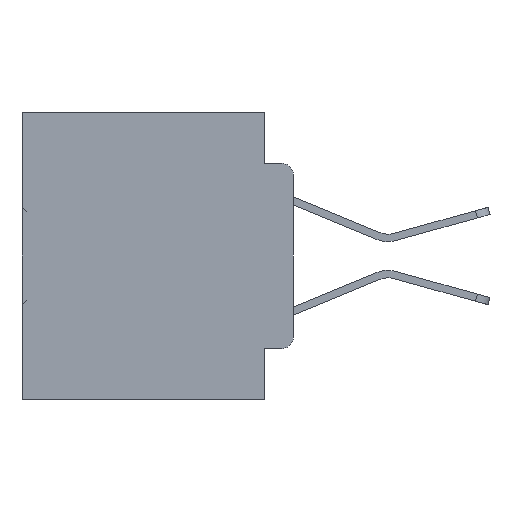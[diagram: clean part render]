
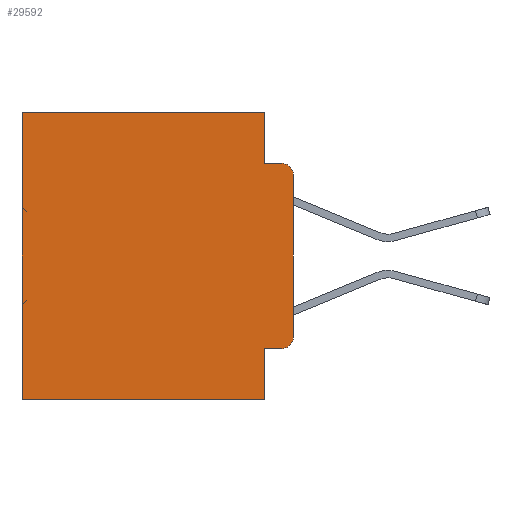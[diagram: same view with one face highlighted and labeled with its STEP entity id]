
A CAD part, left-side view. The second image highlights one B-rep face of the part: STEP entity #29592.
In plain terms, the highlighted planar face has unit normal (-1, 0, 0).
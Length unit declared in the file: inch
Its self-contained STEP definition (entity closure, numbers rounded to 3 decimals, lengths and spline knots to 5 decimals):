
#120 = DIRECTION ( 'NONE',  ( 0., 0., -1. ) ) ;
#474 = DIRECTION ( 'NONE',  ( 0., 1., 0. ) ) ;
#1241 = CARTESIAN_POINT ( 'NONE',  ( 0.298, 0.051, 0. ) ) ;
#1814 = CARTESIAN_POINT ( 'NONE',  ( 0.298, 0., 0. ) ) ;
#1868 = CARTESIAN_POINT ( 'NONE',  ( 0.298, 0.02, -0.3915 ) ) ;
#2194 = CIRCLE ( 'NONE', #7619, 0.02 ) ;
#2796 = EDGE_CURVE ( 'NONE', #21995, #24222, #34332, .T. ) ;
#3744 = LINE ( 'NONE', #35566, #21834 ) ;
#3917 = DIRECTION ( 'NONE',  ( 0., -1., 0. ) ) ;
#4084 = DIRECTION ( 'NONE',  ( -1., 0., 0. ) ) ;
#4510 = LINE ( 'NONE', #27494, #24777 ) ;
#5213 = CARTESIAN_POINT ( 'NONE',  ( 0.298, 0.473, 0. ) ) ;
#5308 = DIRECTION ( 'NONE',  ( 0., 0., -1. ) ) ;
#5920 = DIRECTION ( 'NONE',  ( 0., 1., 0. ) ) ;
#6884 = FACE_OUTER_BOUND ( 'NONE', #13854, .T. ) ;
#7331 = AXIS2_PLACEMENT_3D ( 'NONE', #1814, #30416, #13293 ) ;
#7619 = AXIS2_PLACEMENT_3D ( 'NONE', #15950, #4084, #36111 ) ;
#8648 = VERTEX_POINT ( 'NONE', #34553 ) ;
#11199 = CARTESIAN_POINT ( 'NONE',  ( 0.298, 0., -0.3915 ) ) ;
#11206 = EDGE_CURVE ( 'NONE', #33371, #8648, #17045, .T. ) ;
#11445 = CARTESIAN_POINT ( 'NONE',  ( 0.298, 0.051, -0.4115 ) ) ;
#11586 = EDGE_CURVE ( 'NONE', #36654, #33371, #28913, .T. ) ;
#12088 = ORIENTED_EDGE ( 'NONE', *, *, #11206, .T. ) ;
#12143 = ORIENTED_EDGE ( 'NONE', *, *, #11586, .T. ) ;
#12160 = VECTOR ( 'NONE', #5920, 39.37008 ) ;
#13293 = DIRECTION ( 'NONE',  ( 0., 0., -1. ) ) ;
#13363 = EDGE_CURVE ( 'NONE', #26483, #35936, #26423, .T. ) ;
#13854 = EDGE_LOOP ( 'NONE', ( #20688, #20316, #27046, #24259, #12143, #12088, #21964, #13902, #32856, #25086 ) ) ;
#13902 = ORIENTED_EDGE ( 'NONE', *, *, #2796, .F. ) ;
#14044 = CARTESIAN_POINT ( 'NONE',  ( 0.298, 0.473, 0. ) ) ;
#14551 = LINE ( 'NONE', #31704, #25005 ) ;
#14837 = VECTOR ( 'NONE', #34196, 39.37008 ) ;
#15950 = CARTESIAN_POINT ( 'NONE',  ( 0.298, 0.02, -0.1085 ) ) ;
#17043 = LINE ( 'NONE', #29102, #37125 ) ;
#17045 = LINE ( 'NONE', #14044, #14837 ) ;
#18146 = EDGE_CURVE ( 'NONE', #27950, #18705, #21348, .T. ) ;
#18705 = VERTEX_POINT ( 'NONE', #11199 ) ;
#19619 = VECTOR ( 'NONE', #28685, 39.37008 ) ;
#20316 = ORIENTED_EDGE ( 'NONE', *, *, #36227, .T. ) ;
#20688 = ORIENTED_EDGE ( 'NONE', *, *, #35152, .F. ) ;
#20869 = VECTOR ( 'NONE', #5308, 39.37008 ) ;
#21348 = CIRCLE ( 'NONE', #30350, 0.02 ) ;
#21834 = VECTOR ( 'NONE', #3917, 39.37008 ) ;
#21964 = ORIENTED_EDGE ( 'NONE', *, *, #29976, .F. ) ;
#21995 = VERTEX_POINT ( 'NONE', #11445 ) ;
#22677 = DIRECTION ( 'NONE',  ( 0., 0., -1. ) ) ;
#24222 = VERTEX_POINT ( 'NONE', #34350 ) ;
#24259 = ORIENTED_EDGE ( 'NONE', *, *, #35663, .F. ) ;
#24777 = VECTOR ( 'NONE', #474, 39.37008 ) ;
#25005 = VECTOR ( 'NONE', #22677, 39.37008 ) ;
#25086 = ORIENTED_EDGE ( 'NONE', *, *, #18146, .T. ) ;
#25589 = CARTESIAN_POINT ( 'NONE',  ( 0.298, 0.051, -0.0885 ) ) ;
#25859 = CARTESIAN_POINT ( 'NONE',  ( 0.298, 0.051, -0.0885 ) ) ;
#25896 = CARTESIAN_POINT ( 'NONE',  ( 0.298, 0., 0. ) ) ;
#26423 = LINE ( 'NONE', #25859, #19619 ) ;
#26483 = VERTEX_POINT ( 'NONE', #25589 ) ;
#27046 = ORIENTED_EDGE ( 'NONE', *, *, #13363, .F. ) ;
#27269 = DIRECTION ( 'NONE',  ( -1., 0., 0. ) ) ;
#27494 = CARTESIAN_POINT ( 'NONE',  ( 0.298, 0., -0.5 ) ) ;
#27648 = DIRECTION ( 'NONE',  ( 0., 0., -1. ) ) ;
#27950 = VERTEX_POINT ( 'NONE', #36681 ) ;
#28685 = DIRECTION ( 'NONE',  ( 0., -1., 0. ) ) ;
#28913 = LINE ( 'NONE', #25896, #12160 ) ;
#29102 = CARTESIAN_POINT ( 'NONE',  ( 0.298, 0., 0. ) ) ;
#29493 = PLANE ( 'NONE',  #7331 ) ;
#29592 = ADVANCED_FACE ( 'NONE', ( #6884 ), #29493, .F. ) ;
#29720 = CARTESIAN_POINT ( 'NONE',  ( 0.298, 0., -0.1085 ) ) ;
#29976 = EDGE_CURVE ( 'NONE', #24222, #8648, #4510, .T. ) ;
#30350 = AXIS2_PLACEMENT_3D ( 'NONE', #1868, #27269, #27648 ) ;
#30390 = VERTEX_POINT ( 'NONE', #29720 ) ;
#30416 = DIRECTION ( 'NONE',  ( 1., 0., 0. ) ) ;
#30420 = EDGE_CURVE ( 'NONE', #21995, #27950, #3744, .T. ) ;
#31053 = CARTESIAN_POINT ( 'NONE',  ( 0.298, 0.02, -0.0885 ) ) ;
#31704 = CARTESIAN_POINT ( 'NONE',  ( 0.298, 0.051, 0. ) ) ;
#32856 = ORIENTED_EDGE ( 'NONE', *, *, #30420, .T. ) ;
#33371 = VERTEX_POINT ( 'NONE', #5213 ) ;
#34196 = DIRECTION ( 'NONE',  ( 0., 0., -1. ) ) ;
#34332 = LINE ( 'NONE', #36411, #20869 ) ;
#34350 = CARTESIAN_POINT ( 'NONE',  ( 0.298, 0.051, -0.5 ) ) ;
#34553 = CARTESIAN_POINT ( 'NONE',  ( 0.298, 0.473, -0.5 ) ) ;
#35152 = EDGE_CURVE ( 'NONE', #30390, #18705, #17043, .T. ) ;
#35566 = CARTESIAN_POINT ( 'NONE',  ( 0.298, 0.051, -0.4115 ) ) ;
#35663 = EDGE_CURVE ( 'NONE', #36654, #26483, #14551, .T. ) ;
#35936 = VERTEX_POINT ( 'NONE', #31053 ) ;
#36111 = DIRECTION ( 'NONE',  ( 0., 0., -1. ) ) ;
#36227 = EDGE_CURVE ( 'NONE', #30390, #35936, #2194, .T. ) ;
#36411 = CARTESIAN_POINT ( 'NONE',  ( 0.298, 0.051, 0. ) ) ;
#36654 = VERTEX_POINT ( 'NONE', #1241 ) ;
#36681 = CARTESIAN_POINT ( 'NONE',  ( 0.298, 0.02, -0.4115 ) ) ;
#37125 = VECTOR ( 'NONE', #120, 39.37008 ) ;
